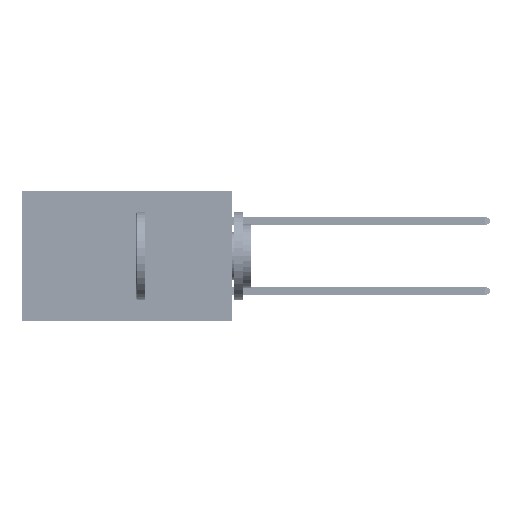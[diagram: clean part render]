
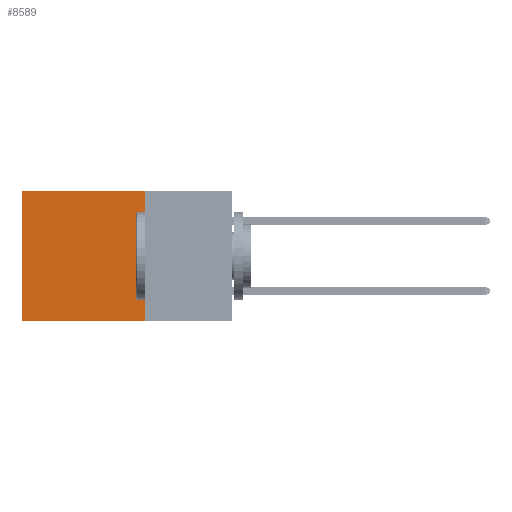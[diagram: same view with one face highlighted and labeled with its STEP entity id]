
A CAD part, left-side view. The second image highlights one B-rep face of the part: STEP entity #8589.
In plain terms, the highlighted planar face has unit normal (-1, 0, 0).
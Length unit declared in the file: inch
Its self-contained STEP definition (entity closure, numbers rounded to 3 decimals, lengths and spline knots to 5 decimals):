
#3275 = CARTESIAN_POINT ( 'NONE',  ( 0.2875, 0.6, 0. ) ) ;
#3603 = DIRECTION ( 'NONE',  ( 0., 0., -1. ) ) ;
#4862 = PLANE ( 'NONE',  #7934 ) ;
#6521 = DIRECTION ( 'NONE',  ( 0., 0., -1. ) ) ;
#6889 = EDGE_CURVE ( 'NONE', #42479, #13458, #22234, .T. ) ;
#7934 = AXIS2_PLACEMENT_3D ( 'NONE', #23789, #42299, #8669 ) ;
#8589 = ADVANCED_FACE ( 'NONE', ( #36151 ), #4862, .F. ) ;
#8669 = DIRECTION ( 'NONE',  ( 0., 0., -1. ) ) ;
#9020 = CARTESIAN_POINT ( 'NONE',  ( 0.2875, 0.25, -0.37 ) ) ;
#9352 = CARTESIAN_POINT ( 'NONE',  ( 0.2875, 0.25, 0. ) ) ;
#9637 = VECTOR ( 'NONE', #29364, 39.37008 ) ;
#11326 = EDGE_CURVE ( 'NONE', #42479, #48326, #28628, .T. ) ;
#12269 = LINE ( 'NONE', #33789, #31172 ) ;
#13458 = VERTEX_POINT ( 'NONE', #9020 ) ;
#17944 = CARTESIAN_POINT ( 'NONE',  ( 0.2875, 0.25, -0.37 ) ) ;
#18475 = EDGE_CURVE ( 'NONE', #13458, #27538, #20934, .T. ) ;
#20934 = LINE ( 'NONE', #17944, #9637 ) ;
#21705 = ORIENTED_EDGE ( 'NONE', *, *, #6889, .F. ) ;
#22234 = LINE ( 'NONE', #29189, #23435 ) ;
#23435 = VECTOR ( 'NONE', #6521, 39.37008 ) ;
#23789 = CARTESIAN_POINT ( 'NONE',  ( 0.2875, 0.25, 0. ) ) ;
#27538 = VERTEX_POINT ( 'NONE', #35064 ) ;
#27672 = CARTESIAN_POINT ( 'NONE',  ( 0.2875, 0.25, 0. ) ) ;
#28628 = LINE ( 'NONE', #9352, #40794 ) ;
#29189 = CARTESIAN_POINT ( 'NONE',  ( 0.2875, 0.25, 0. ) ) ;
#29364 = DIRECTION ( 'NONE',  ( 0., 1., 0. ) ) ;
#30797 = EDGE_LOOP ( 'NONE', ( #48172, #37262, #21705, #39065 ) ) ;
#31172 = VECTOR ( 'NONE', #3603, 39.37008 ) ;
#33789 = CARTESIAN_POINT ( 'NONE',  ( 0.2875, 0.6, 0. ) ) ;
#34741 = EDGE_CURVE ( 'NONE', #48326, #27538, #12269, .T. ) ;
#35064 = CARTESIAN_POINT ( 'NONE',  ( 0.2875, 0.6, -0.37 ) ) ;
#35690 = DIRECTION ( 'NONE',  ( 0., 1., 0. ) ) ;
#36151 = FACE_OUTER_BOUND ( 'NONE', #30797, .T. ) ;
#37262 = ORIENTED_EDGE ( 'NONE', *, *, #18475, .F. ) ;
#39065 = ORIENTED_EDGE ( 'NONE', *, *, #11326, .T. ) ;
#40794 = VECTOR ( 'NONE', #35690, 39.37008 ) ;
#42299 = DIRECTION ( 'NONE',  ( 1., 0., 0. ) ) ;
#42479 = VERTEX_POINT ( 'NONE', #27672 ) ;
#48172 = ORIENTED_EDGE ( 'NONE', *, *, #34741, .T. ) ;
#48326 = VERTEX_POINT ( 'NONE', #3275 ) ;
